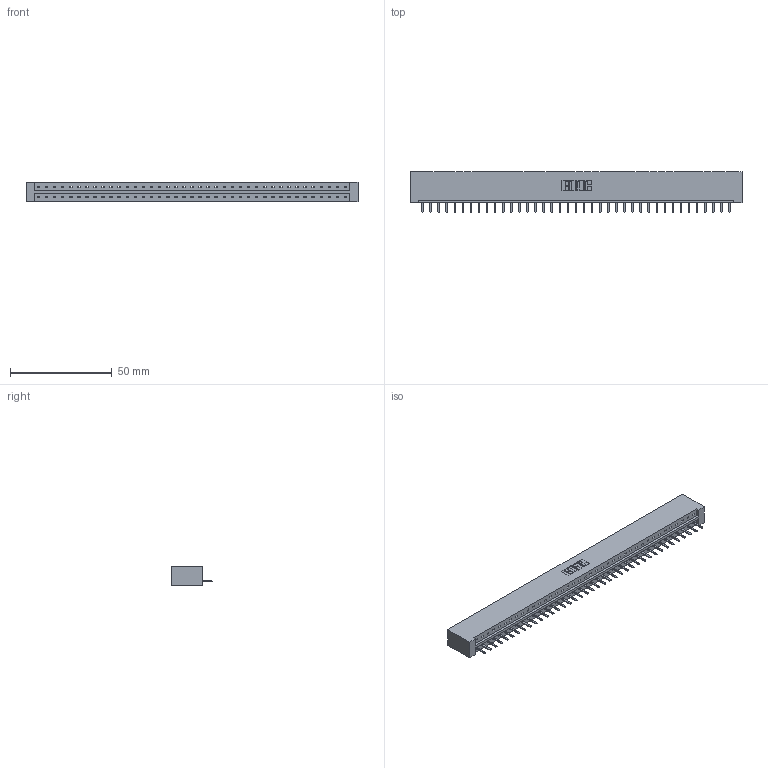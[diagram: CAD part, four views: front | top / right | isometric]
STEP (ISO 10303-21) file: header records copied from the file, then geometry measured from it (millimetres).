
FILE_DESCRIPTION (( 'STEP AP203' ), '1' );
FILE_NAME ('333-039-520-101.STEP', '2018-08-03T12:26:03', ( '' ), ( '' ), 'SwSTEP 2.0', 'SolidWorks 2016', '' );
FILE_SCHEMA (( 'CONFIG_CONTROL_DESIGN' ));
Length unit declared in the file: inch
Products named in the file (3): 333 Part_Lugless; 345-292-001_345-293-120; 333-039-520-101
Assembly tree (40 placements, depth 2):
  333-039-520-101
    333 Part_Lugless
    345-292-001_345-293-120  x39
Bounding box: 162.79 x 20.02 x 9.4 mm (x, y, z)
Volume: 16855.9 mm3; surface area: 17781.2 mm2
Topology: 40 solids, 40 shells, 2524 faces, 7463 edges, 4870 vertices
Faces by surface type: plane 1782, cylinder 742
Entity records: 24067 total; most frequent: CARTESIAN_POINT 4171, ORIENTED_EDGE 4134, DIRECTION 3505, EDGE_CURVE 2067, VECTOR 1943, LINE 1943, VERTEX_POINT 1374, AXIS2_PLACEMENT_3D 781
